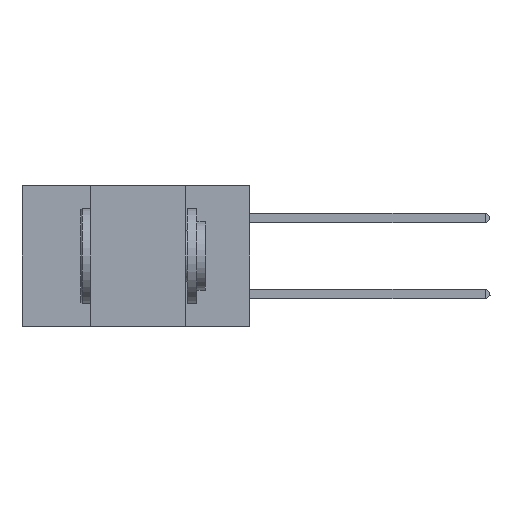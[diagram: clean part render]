
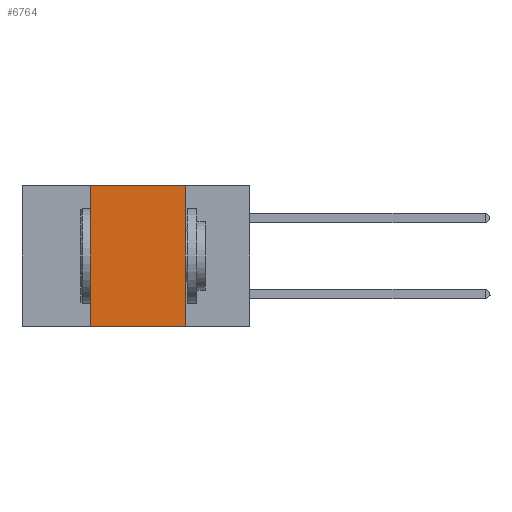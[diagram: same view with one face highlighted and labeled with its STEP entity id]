
A CAD part, left-side view. The second image highlights one B-rep face of the part: STEP entity #6764.
In plain terms, the highlighted planar face has unit normal (-1, 0, 0).
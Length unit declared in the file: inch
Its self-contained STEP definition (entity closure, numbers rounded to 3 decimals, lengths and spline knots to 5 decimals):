
#582 = VERTEX_POINT ( 'NONE', #8529 ) ;
#711 = CARTESIAN_POINT ( 'NONE',  ( 0., 0.42, 0. ) ) ;
#715 = ORIENTED_EDGE ( 'NONE', *, *, #13233, .F. ) ;
#745 = DIRECTION ( 'NONE',  ( 0., 0., -1. ) ) ;
#1035 = PLANE ( 'NONE',  #11447 ) ;
#3565 = ORIENTED_EDGE ( 'NONE', *, *, #19522, .T. ) ;
#4245 = CARTESIAN_POINT ( 'NONE',  ( 0., 0.17, 0. ) ) ;
#4258 = CARTESIAN_POINT ( 'NONE',  ( 0., 0.6, -0.37 ) ) ;
#4534 = VERTEX_POINT ( 'NONE', #711 ) ;
#6362 = CARTESIAN_POINT ( 'NONE',  ( 0., 0.6, 0. ) ) ;
#6764 = ADVANCED_FACE ( 'NONE', ( #16038 ), #1035, .F. ) ;
#7850 = CARTESIAN_POINT ( 'NONE',  ( 0., 0.17, -0.37 ) ) ;
#7998 = LINE ( 'NONE', #22562, #17022 ) ;
#8529 = CARTESIAN_POINT ( 'NONE',  ( 0., 0.42, -0.37 ) ) ;
#9062 = EDGE_CURVE ( 'NONE', #582, #4534, #18147, .T. ) ;
#10076 = DIRECTION ( 'NONE',  ( 0., 0., -1. ) ) ;
#10414 = CARTESIAN_POINT ( 'NONE',  ( 0., 0.17, 0. ) ) ;
#11447 = AXIS2_PLACEMENT_3D ( 'NONE', #6362, #13501, #10076 ) ;
#12905 = ORIENTED_EDGE ( 'NONE', *, *, #17805, .F. ) ;
#13233 = EDGE_CURVE ( 'NONE', #17491, #15812, #22297, .T. ) ;
#13501 = DIRECTION ( 'NONE',  ( 1., 0., 0. ) ) ;
#15790 = DIRECTION ( 'NONE',  ( 0., -1., 0. ) ) ;
#15812 = VERTEX_POINT ( 'NONE', #7850 ) ;
#16038 = FACE_OUTER_BOUND ( 'NONE', #17930, .T. ) ;
#16103 = VECTOR ( 'NONE', #16493, 39.37008 ) ;
#16493 = DIRECTION ( 'NONE',  ( 0., -1., 0. ) ) ;
#17022 = VECTOR ( 'NONE', #15790, 39.37008 ) ;
#17491 = VERTEX_POINT ( 'NONE', #10414 ) ;
#17768 = ORIENTED_EDGE ( 'NONE', *, *, #9062, .F. ) ;
#17805 = EDGE_CURVE ( 'NONE', #4534, #17491, #7998, .T. ) ;
#17930 = EDGE_LOOP ( 'NONE', ( #715, #12905, #17768, #3565 ) ) ;
#18147 = LINE ( 'NONE', #22565, #22068 ) ;
#19418 = LINE ( 'NONE', #4258, #16103 ) ;
#19522 = EDGE_CURVE ( 'NONE', #582, #15812, #19418, .T. ) ;
#20647 = DIRECTION ( 'NONE',  ( 0., 0., 1. ) ) ;
#21449 = VECTOR ( 'NONE', #745, 39.37008 ) ;
#22068 = VECTOR ( 'NONE', #20647, 39.37008 ) ;
#22297 = LINE ( 'NONE', #4245, #21449 ) ;
#22562 = CARTESIAN_POINT ( 'NONE',  ( 0., 0.6, 0. ) ) ;
#22565 = CARTESIAN_POINT ( 'NONE',  ( 0., 0.42, 0. ) ) ;
